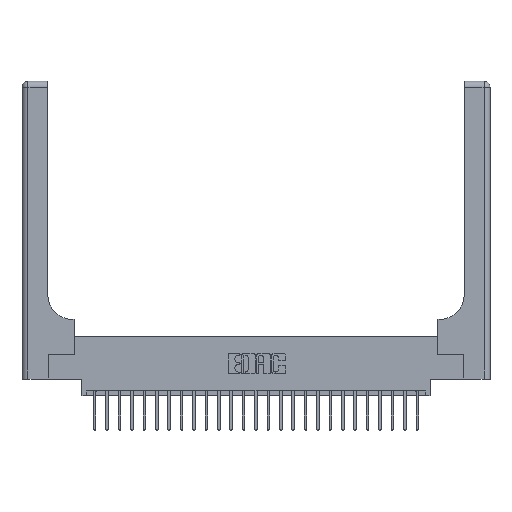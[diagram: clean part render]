
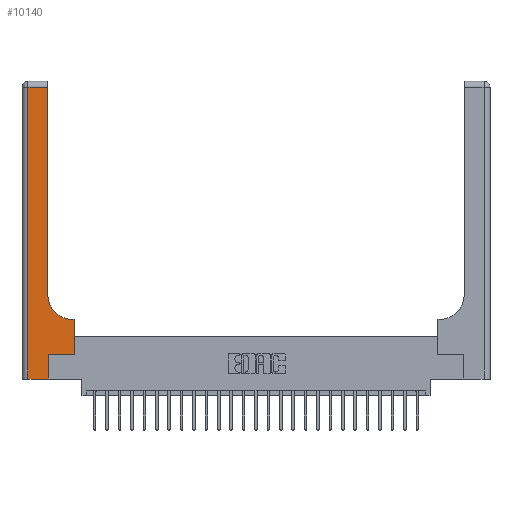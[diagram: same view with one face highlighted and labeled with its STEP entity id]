
A CAD part, top view. The second image highlights one B-rep face of the part: STEP entity #10140.
In plain terms, the highlighted planar face has unit normal (0, 0, 1).
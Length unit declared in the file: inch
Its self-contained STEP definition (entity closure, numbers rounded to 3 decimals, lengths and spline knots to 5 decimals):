
#312 = VECTOR ( 'NONE', #13317, 39.37008 ) ;
#497 = DIRECTION ( 'NONE',  ( 0., 0., -1. ) ) ;
#777 = CARTESIAN_POINT ( 'NONE',  ( 0.26, 0.85, 0.37 ) ) ;
#1025 = VERTEX_POINT ( 'NONE', #18382 ) ;
#1463 = CARTESIAN_POINT ( 'NONE',  ( 0.528, 0.25, 0.37 ) ) ;
#1621 = LINE ( 'NONE', #7033, #11244 ) ;
#1815 = ORIENTED_EDGE ( 'NONE', *, *, #11903, .T. ) ;
#1874 = ORIENTED_EDGE ( 'NONE', *, *, #4565, .T. ) ;
#2564 = VECTOR ( 'NONE', #9739, 39.37008 ) ;
#3643 = VERTEX_POINT ( 'NONE', #11392 ) ;
#4565 = EDGE_CURVE ( 'NONE', #11561, #1025, #6528, .T. ) ;
#4622 = ORIENTED_EDGE ( 'NONE', *, *, #16711, .T. ) ;
#5528 = EDGE_CURVE ( 'NONE', #15942, #23349, #17365, .T. ) ;
#6054 = AXIS2_PLACEMENT_3D ( 'NONE', #10014, #23562, #12001 ) ;
#6064 = VERTEX_POINT ( 'NONE', #13750 ) ;
#6528 = LINE ( 'NONE', #14250, #21347 ) ;
#6680 = LINE ( 'NONE', #7475, #312 ) ;
#6918 = VERTEX_POINT ( 'NONE', #1463 ) ;
#7033 = CARTESIAN_POINT ( 'NONE',  ( 0.06, 3., 0.37 ) ) ;
#7108 = DIRECTION ( 'NONE',  ( 0., -1., 0. ) ) ;
#7475 = CARTESIAN_POINT ( 'NONE',  ( 0., 2.94, 0.37 ) ) ;
#8687 = ORIENTED_EDGE ( 'NONE', *, *, #5528, .T. ) ;
#9739 = DIRECTION ( 'NONE',  ( 0., 1., 0. ) ) ;
#9911 = VECTOR ( 'NONE', #20180, 39.37008 ) ;
#10014 = CARTESIAN_POINT ( 'NONE',  ( 0.51, 0.85, 0.37 ) ) ;
#10140 = ADVANCED_FACE ( 'NONE', ( #20143 ), #23635, .F. ) ;
#10467 = DIRECTION ( 'NONE',  ( 1., 0., 0. ) ) ;
#11244 = VECTOR ( 'NONE', #7108, 39.37008 ) ;
#11392 = CARTESIAN_POINT ( 'NONE',  ( 0.51, 0.6, 0.37 ) ) ;
#11427 = AXIS2_PLACEMENT_3D ( 'NONE', #19781, #497, #14025 ) ;
#11496 = EDGE_LOOP ( 'NONE', ( #8687, #12982, #18589, #1874, #4622, #1815, #21501, #23699, #11867 ) ) ;
#11561 = VERTEX_POINT ( 'NONE', #20932 ) ;
#11867 = ORIENTED_EDGE ( 'NONE', *, *, #18140, .T. ) ;
#11870 = VECTOR ( 'NONE', #19859, 39.37008 ) ;
#11903 = EDGE_CURVE ( 'NONE', #24993, #6918, #24633, .T. ) ;
#12001 = DIRECTION ( 'NONE',  ( 1., 0., 0. ) ) ;
#12626 = CARTESIAN_POINT ( 'NONE',  ( 0.528, 0.25, 0.37 ) ) ;
#12982 = ORIENTED_EDGE ( 'NONE', *, *, #22021, .T. ) ;
#13092 = VERTEX_POINT ( 'NONE', #13323 ) ;
#13317 = DIRECTION ( 'NONE',  ( -1., 0., 0. ) ) ;
#13323 = CARTESIAN_POINT ( 'NONE',  ( 0.528, 0.6, 0.37 ) ) ;
#13750 = CARTESIAN_POINT ( 'NONE',  ( 0.06, 2.94, 0.37 ) ) ;
#14025 = DIRECTION ( 'NONE',  ( -1., 0., 0. ) ) ;
#14250 = CARTESIAN_POINT ( 'NONE',  ( 0., 0., 0.37 ) ) ;
#14487 = VECTOR ( 'NONE', #24186, 39.37008 ) ;
#14637 = EDGE_CURVE ( 'NONE', #13092, #3643, #17042, .T. ) ;
#15714 = LINE ( 'NONE', #12626, #14487 ) ;
#15912 = CARTESIAN_POINT ( 'NONE',  ( 0.265, 0.25, 0.37 ) ) ;
#15942 = VERTEX_POINT ( 'NONE', #777 ) ;
#16367 = CARTESIAN_POINT ( 'NONE',  ( 0.265, 0.25, 0.37 ) ) ;
#16412 = CARTESIAN_POINT ( 'NONE',  ( 0.265, 0., 0.37 ) ) ;
#16711 = EDGE_CURVE ( 'NONE', #1025, #24993, #20246, .T. ) ;
#17042 = LINE ( 'NONE', #23633, #11870 ) ;
#17184 = EDGE_CURVE ( 'NONE', #6918, #13092, #15714, .T. ) ;
#17365 = LINE ( 'NONE', #17494, #2564 ) ;
#17494 = CARTESIAN_POINT ( 'NONE',  ( 0.26, 3., 0.37 ) ) ;
#18140 = EDGE_CURVE ( 'NONE', #3643, #15942, #20171, .T. ) ;
#18382 = CARTESIAN_POINT ( 'NONE',  ( 0.265, 0., 0.37 ) ) ;
#18589 = ORIENTED_EDGE ( 'NONE', *, *, #20729, .T. ) ;
#18598 = CARTESIAN_POINT ( 'NONE',  ( 0.26, 2.94, 0.37 ) ) ;
#18945 = VECTOR ( 'NONE', #10467, 39.37008 ) ;
#19781 = CARTESIAN_POINT ( 'NONE',  ( 0., 3., 0.37 ) ) ;
#19859 = DIRECTION ( 'NONE',  ( -1., 0., 0. ) ) ;
#20067 = DIRECTION ( 'NONE',  ( 1., 0., 0. ) ) ;
#20143 = FACE_OUTER_BOUND ( 'NONE', #11496, .T. ) ;
#20171 = CIRCLE ( 'NONE', #6054, 0.25 ) ;
#20180 = DIRECTION ( 'NONE',  ( 0., 1., 0. ) ) ;
#20246 = LINE ( 'NONE', #16412, #9911 ) ;
#20729 = EDGE_CURVE ( 'NONE', #6064, #11561, #1621, .T. ) ;
#20932 = CARTESIAN_POINT ( 'NONE',  ( 0.06, 0., 0.37 ) ) ;
#21347 = VECTOR ( 'NONE', #20067, 39.37008 ) ;
#21501 = ORIENTED_EDGE ( 'NONE', *, *, #17184, .T. ) ;
#22021 = EDGE_CURVE ( 'NONE', #23349, #6064, #6680, .T. ) ;
#23349 = VERTEX_POINT ( 'NONE', #18598 ) ;
#23562 = DIRECTION ( 'NONE',  ( 0., 0., -1. ) ) ;
#23633 = CARTESIAN_POINT ( 'NONE',  ( 0.26, 0.6, 0.37 ) ) ;
#23635 = PLANE ( 'NONE',  #11427 ) ;
#23699 = ORIENTED_EDGE ( 'NONE', *, *, #14637, .T. ) ;
#24186 = DIRECTION ( 'NONE',  ( 0., 1., 0. ) ) ;
#24633 = LINE ( 'NONE', #16367, #18945 ) ;
#24993 = VERTEX_POINT ( 'NONE', #15912 ) ;
